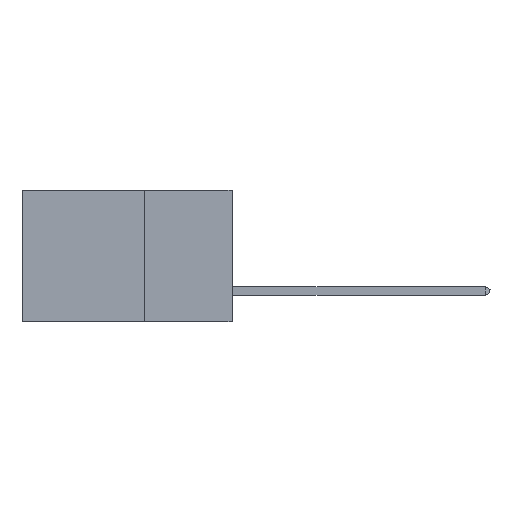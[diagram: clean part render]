
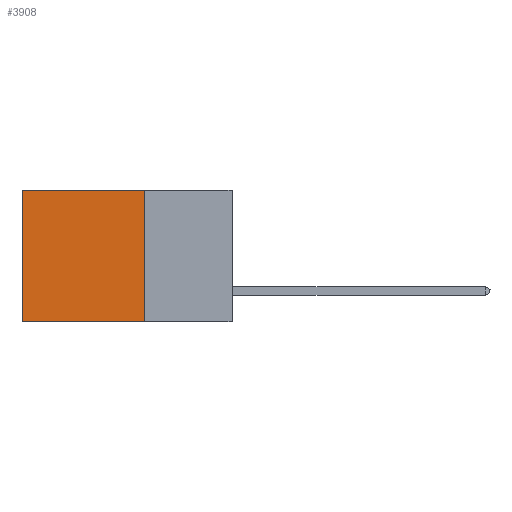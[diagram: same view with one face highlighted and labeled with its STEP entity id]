
A CAD part, left-side view. The second image highlights one B-rep face of the part: STEP entity #3908.
In plain terms, the highlighted planar face has unit normal (-1, 0, 0).
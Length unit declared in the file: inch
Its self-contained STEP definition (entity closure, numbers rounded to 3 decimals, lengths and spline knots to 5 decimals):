
#556 = ORIENTED_EDGE ( 'NONE', *, *, #17976, .T. ) ;
#596 = EDGE_CURVE ( 'NONE', #16223, #4568, #3905, .T. ) ;
#699 = LINE ( 'NONE', #17140, #4631 ) ;
#702 = DIRECTION ( 'NONE',  ( 0., 0., -1. ) ) ;
#2297 = CARTESIAN_POINT ( 'NONE',  ( 0.2875, 0.25, -0.375 ) ) ;
#2850 = DIRECTION ( 'NONE',  ( 0., 0., -1. ) ) ;
#2928 = CARTESIAN_POINT ( 'NONE',  ( 0.2875, 0.25, 0. ) ) ;
#3905 = LINE ( 'NONE', #19050, #11307 ) ;
#3908 = ADVANCED_FACE ( 'NONE', ( #14854 ), #9504, .F. ) ;
#4323 = VECTOR ( 'NONE', #15656, 39.37008 ) ;
#4568 = VERTEX_POINT ( 'NONE', #8911 ) ;
#4631 = VECTOR ( 'NONE', #15706, 39.37008 ) ;
#5241 = CARTESIAN_POINT ( 'NONE',  ( 0.2875, 0.25, -0.375 ) ) ;
#5777 = EDGE_CURVE ( 'NONE', #13034, #4568, #699, .T. ) ;
#7095 = ORIENTED_EDGE ( 'NONE', *, *, #13760, .F. ) ;
#7215 = LINE ( 'NONE', #17699, #7677 ) ;
#7677 = VECTOR ( 'NONE', #10340, 39.37008 ) ;
#8074 = CARTESIAN_POINT ( 'NONE',  ( 0.2875, 0.25, -0.375 ) ) ;
#8425 = ORIENTED_EDGE ( 'NONE', *, *, #5777, .F. ) ;
#8911 = CARTESIAN_POINT ( 'NONE',  ( 0.2875, 0.6, -0.375 ) ) ;
#9504 = PLANE ( 'NONE',  #16314 ) ;
#10340 = DIRECTION ( 'NONE',  ( 0., 1., 0. ) ) ;
#10580 = LINE ( 'NONE', #2297, #4323 ) ;
#11307 = VECTOR ( 'NONE', #2850, 39.37008 ) ;
#12449 = DIRECTION ( 'NONE',  ( 1., 0., 0. ) ) ;
#13034 = VERTEX_POINT ( 'NONE', #5241 ) ;
#13216 = VERTEX_POINT ( 'NONE', #2928 ) ;
#13760 = EDGE_CURVE ( 'NONE', #13216, #13034, #10580, .T. ) ;
#14854 = FACE_OUTER_BOUND ( 'NONE', #15813, .T. ) ;
#15101 = CARTESIAN_POINT ( 'NONE',  ( 0.2875, 0.6, 0. ) ) ;
#15656 = DIRECTION ( 'NONE',  ( 0., 0., -1. ) ) ;
#15706 = DIRECTION ( 'NONE',  ( 0., 1., 0. ) ) ;
#15813 = EDGE_LOOP ( 'NONE', ( #18729, #8425, #7095, #556 ) ) ;
#16223 = VERTEX_POINT ( 'NONE', #15101 ) ;
#16314 = AXIS2_PLACEMENT_3D ( 'NONE', #8074, #12449, #702 ) ;
#17140 = CARTESIAN_POINT ( 'NONE',  ( 0.2875, 0.25, -0.375 ) ) ;
#17699 = CARTESIAN_POINT ( 'NONE',  ( 0.2875, 0.25, 0. ) ) ;
#17976 = EDGE_CURVE ( 'NONE', #13216, #16223, #7215, .T. ) ;
#18729 = ORIENTED_EDGE ( 'NONE', *, *, #596, .T. ) ;
#19050 = CARTESIAN_POINT ( 'NONE',  ( 0.2875, 0.6, -0.375 ) ) ;
